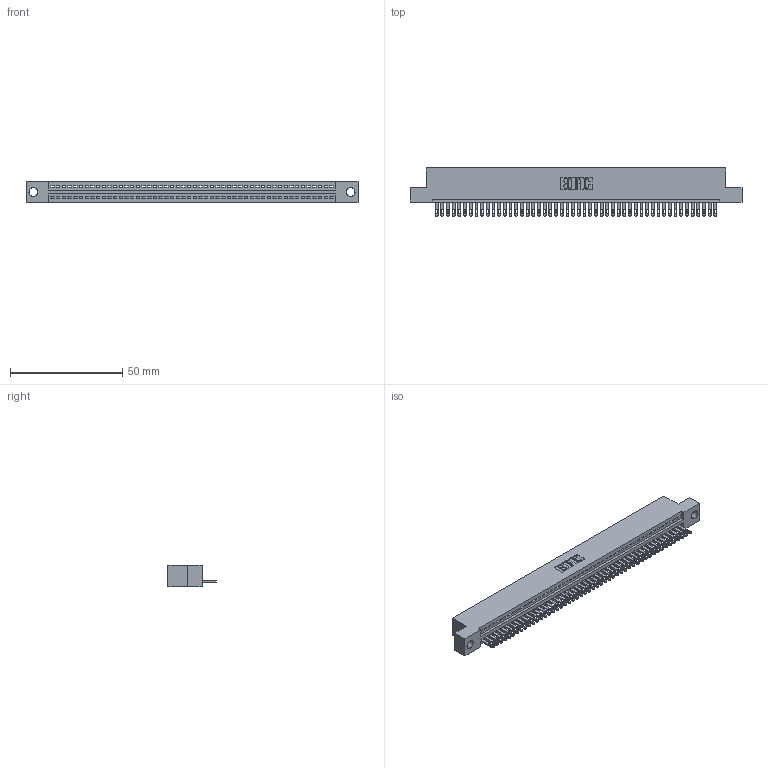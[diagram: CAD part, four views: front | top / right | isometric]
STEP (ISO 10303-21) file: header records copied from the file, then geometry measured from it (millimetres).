
FILE_DESCRIPTION (( 'STEP AP203' ), '1' );
FILE_NAME ('895-050-500-104.STEP', '2020-09-27T08:39:15', ( '' ), ( '' ), 'SwSTEP 2.0', 'SolidWorks 2020', '' );
FILE_SCHEMA (( 'CONFIG_CONTROL_DESIGN' ));
Length unit declared in the file: inch
Products named in the file (3): 845 Part_Flush Mounting Lugs - 0.156 Dia-TH; 895-050-500-104; 345-292-001_345-293-100
Assembly tree (51 placements, depth 2):
  895-050-500-104
    845 Part_Flush Mounting Lugs - 0.156 Dia-TH
    345-292-001_345-293-100  x50
Bounding box: 148.21 x 21.51 x 9.4 mm (x, y, z)
Volume: 14085.7 mm3; surface area: 18748.3 mm2
Topology: 51 solids, 51 shells, 2826 faces, 8741 edges, 5826 vertices
Faces by surface type: plane 1780, cylinder 1046
Entity records: 36487 total; most frequent: CARTESIAN_POINT 6326, ORIENTED_EDGE 6310, DIRECTION 5515, EDGE_CURVE 3155, VECTOR 2819, LINE 2819, VERTEX_POINT 2102, AXIS2_PLACEMENT_3D 1348
